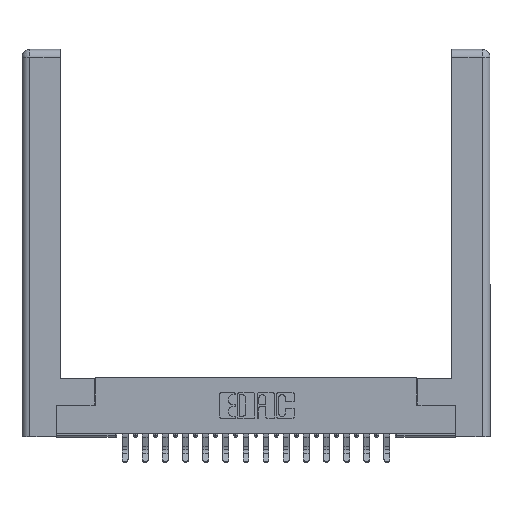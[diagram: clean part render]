
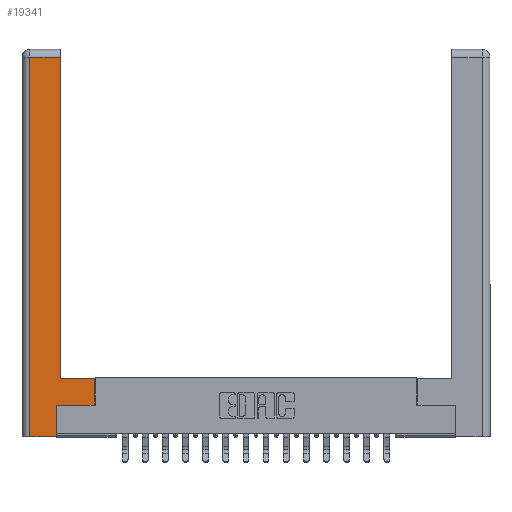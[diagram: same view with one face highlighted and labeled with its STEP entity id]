
A CAD part, top view. The second image highlights one B-rep face of the part: STEP entity #19341.
In plain terms, the highlighted planar face has unit normal (0, 0, 1).
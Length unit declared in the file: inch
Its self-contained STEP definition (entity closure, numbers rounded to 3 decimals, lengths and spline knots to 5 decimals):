
#460 = CARTESIAN_POINT ( 'NONE',  ( 0.0615, 2.94, 0. ) ) ;
#506 = ORIENTED_EDGE ( 'NONE', *, *, #12631, .T. ) ;
#927 = LINE ( 'NONE', #1544, #5058 ) ;
#1544 = CARTESIAN_POINT ( 'NONE',  ( 0.565, 0.245, 0. ) ) ;
#1968 = EDGE_CURVE ( 'NONE', #18821, #17410, #11142, .T. ) ;
#1983 = DIRECTION ( 'NONE',  ( 0., 1., 0. ) ) ;
#2549 = FACE_OUTER_BOUND ( 'NONE', #10977, .T. ) ;
#2688 = VECTOR ( 'NONE', #6566, 39.37008 ) ;
#2721 = ORIENTED_EDGE ( 'NONE', *, *, #1968, .T. ) ;
#2925 = VECTOR ( 'NONE', #11107, 39.37008 ) ;
#3203 = ORIENTED_EDGE ( 'NONE', *, *, #15748, .T. ) ;
#3440 = ORIENTED_EDGE ( 'NONE', *, *, #3582, .T. ) ;
#3582 = EDGE_CURVE ( 'NONE', #17410, #6820, #6463, .T. ) ;
#3872 = VECTOR ( 'NONE', #15779, 39.37008 ) ;
#3908 = ORIENTED_EDGE ( 'NONE', *, *, #7460, .T. ) ;
#5058 = VECTOR ( 'NONE', #18241, 39.37008 ) ;
#5290 = CARTESIAN_POINT ( 'NONE',  ( 0.265, 0., 0. ) ) ;
#6391 = PLANE ( 'NONE',  #11042 ) ;
#6463 = LINE ( 'NONE', #10717, #3872 ) ;
#6566 = DIRECTION ( 'NONE',  ( -1., 0., 0. ) ) ;
#6596 = LINE ( 'NONE', #21052, #2925 ) ;
#6820 = VERTEX_POINT ( 'NONE', #18798 ) ;
#6911 = ORIENTED_EDGE ( 'NONE', *, *, #13651, .T. ) ;
#7008 = CARTESIAN_POINT ( 'NONE',  ( 0.295, 2.94, 0. ) ) ;
#7028 = DIRECTION ( 'NONE',  ( 1., 0., 0. ) ) ;
#7460 = EDGE_CURVE ( 'NONE', #18344, #12947, #19893, .T. ) ;
#7697 = CARTESIAN_POINT ( 'NONE',  ( 0.565, 0.45, 0. ) ) ;
#7737 = LINE ( 'NONE', #5290, #13939 ) ;
#8552 = CARTESIAN_POINT ( 'NONE',  ( 0.295, 3., 0. ) ) ;
#9406 = DIRECTION ( 'NONE',  ( 0., 1., 0. ) ) ;
#9437 = CARTESIAN_POINT ( 'NONE',  ( 0.265, 0.245, 0. ) ) ;
#10717 = CARTESIAN_POINT ( 'NONE',  ( 0.0615, 0., 0. ) ) ;
#10977 = EDGE_LOOP ( 'NONE', ( #6911, #2721, #3440, #506, #3908, #3203, #14550, #12745 ) ) ;
#10993 = CARTESIAN_POINT ( 'NONE',  ( 0.265, 0.245, 0. ) ) ;
#11042 = AXIS2_PLACEMENT_3D ( 'NONE', #21069, #11126, #16202 ) ;
#11107 = DIRECTION ( 'NONE',  ( 0., 1., 0. ) ) ;
#11126 = DIRECTION ( 'NONE',  ( 0., 0., -1. ) ) ;
#11142 = LINE ( 'NONE', #11873, #14520 ) ;
#11274 = VECTOR ( 'NONE', #9406, 39.37008 ) ;
#11431 = CARTESIAN_POINT ( 'NONE',  ( 0.295, 0.45, 0. ) ) ;
#11490 = LINE ( 'NONE', #11431, #2688 ) ;
#11643 = DIRECTION ( 'NONE',  ( -1., 0., 0. ) ) ;
#11873 = CARTESIAN_POINT ( 'NONE',  ( 0.0615, 2.94, 0. ) ) ;
#12032 = VERTEX_POINT ( 'NONE', #17250 ) ;
#12631 = EDGE_CURVE ( 'NONE', #6820, #18344, #7737, .T. ) ;
#12745 = ORIENTED_EDGE ( 'NONE', *, *, #16190, .T. ) ;
#12947 = VERTEX_POINT ( 'NONE', #9437 ) ;
#13123 = VECTOR ( 'NONE', #1983, 39.37008 ) ;
#13651 = EDGE_CURVE ( 'NONE', #12032, #18821, #14972, .T. ) ;
#13939 = VECTOR ( 'NONE', #7028, 39.37008 ) ;
#14520 = VECTOR ( 'NONE', #11643, 39.37008 ) ;
#14550 = ORIENTED_EDGE ( 'NONE', *, *, #16745, .T. ) ;
#14907 = CARTESIAN_POINT ( 'NONE',  ( 0.565, 0.245, 0. ) ) ;
#14972 = LINE ( 'NONE', #8552, #13123 ) ;
#15748 = EDGE_CURVE ( 'NONE', #12947, #21287, #927, .T. ) ;
#15779 = DIRECTION ( 'NONE',  ( 0., -1., 0. ) ) ;
#16022 = VERTEX_POINT ( 'NONE', #7697 ) ;
#16190 = EDGE_CURVE ( 'NONE', #16022, #12032, #11490, .T. ) ;
#16202 = DIRECTION ( 'NONE',  ( -1., 0., 0. ) ) ;
#16745 = EDGE_CURVE ( 'NONE', #21287, #16022, #6596, .T. ) ;
#17250 = CARTESIAN_POINT ( 'NONE',  ( 0.295, 0.45, 0. ) ) ;
#17410 = VERTEX_POINT ( 'NONE', #460 ) ;
#17874 = CARTESIAN_POINT ( 'NONE',  ( 0.265, 0., 0. ) ) ;
#18241 = DIRECTION ( 'NONE',  ( 1., 0., 0. ) ) ;
#18344 = VERTEX_POINT ( 'NONE', #17874 ) ;
#18798 = CARTESIAN_POINT ( 'NONE',  ( 0.0615, 0., 0. ) ) ;
#18821 = VERTEX_POINT ( 'NONE', #7008 ) ;
#19341 = ADVANCED_FACE ( 'NONE', ( #2549 ), #6391, .F. ) ;
#19893 = LINE ( 'NONE', #10993, #11274 ) ;
#21052 = CARTESIAN_POINT ( 'NONE',  ( 0.565, 0.45, 0. ) ) ;
#21069 = CARTESIAN_POINT ( 'NONE',  ( 0., 0., 0. ) ) ;
#21287 = VERTEX_POINT ( 'NONE', #14907 ) ;
